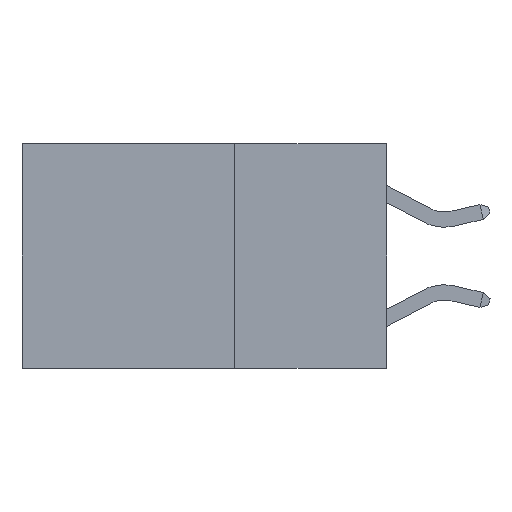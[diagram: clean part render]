
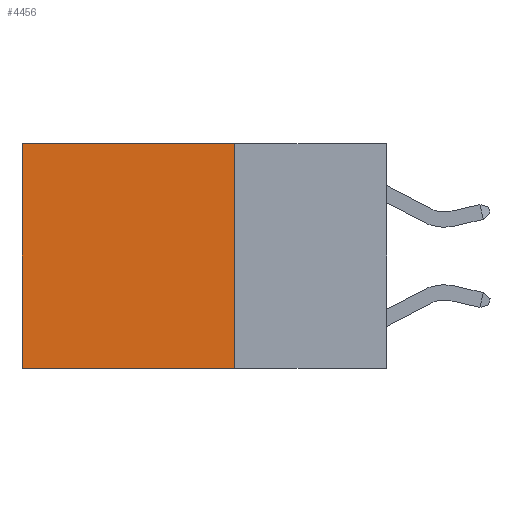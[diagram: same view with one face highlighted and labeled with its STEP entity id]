
A CAD part, left-side view. The second image highlights one B-rep face of the part: STEP entity #4456.
In plain terms, the highlighted planar face has unit normal (-1, 0, 0).
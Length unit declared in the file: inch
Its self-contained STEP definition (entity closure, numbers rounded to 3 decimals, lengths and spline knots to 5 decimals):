
#65 = LINE ( 'NONE', #5386, #7478 ) ;
#236 = CARTESIAN_POINT ( 'NONE',  ( 0.2625, 0.25, 0. ) ) ;
#237 = DIRECTION ( 'NONE',  ( 0., 1., 0. ) ) ;
#862 = PLANE ( 'NONE',  #7459 ) ;
#888 = VERTEX_POINT ( 'NONE', #8403 ) ;
#942 = CARTESIAN_POINT ( 'NONE',  ( 0.2625, 0.25, -0.37 ) ) ;
#1309 = LINE ( 'NONE', #7351, #4073 ) ;
#2309 = CARTESIAN_POINT ( 'NONE',  ( 0.2625, 0.25, 0. ) ) ;
#2523 = VECTOR ( 'NONE', #3492, 39.37008 ) ;
#2684 = FACE_OUTER_BOUND ( 'NONE', #4488, .T. ) ;
#2842 = EDGE_CURVE ( 'NONE', #2978, #7182, #1309, .T. ) ;
#2978 = VERTEX_POINT ( 'NONE', #942 ) ;
#3234 = VECTOR ( 'NONE', #237, 39.37008 ) ;
#3473 = DIRECTION ( 'NONE',  ( 0., 0., -1. ) ) ;
#3492 = DIRECTION ( 'NONE',  ( 0., 0., -1. ) ) ;
#3498 = EDGE_CURVE ( 'NONE', #4253, #2978, #65, .T. ) ;
#3987 = CARTESIAN_POINT ( 'NONE',  ( 0.2625, 0.25, 0. ) ) ;
#4073 = VECTOR ( 'NONE', #5890, 39.37008 ) ;
#4125 = DIRECTION ( 'NONE',  ( 0., 0., -1. ) ) ;
#4253 = VERTEX_POINT ( 'NONE', #236 ) ;
#4313 = ORIENTED_EDGE ( 'NONE', *, *, #6847, .T. ) ;
#4456 = ADVANCED_FACE ( 'NONE', ( #2684 ), #862, .F. ) ;
#4488 = EDGE_LOOP ( 'NONE', ( #4539, #7714, #7367, #4313 ) ) ;
#4539 = ORIENTED_EDGE ( 'NONE', *, *, #6703, .T. ) ;
#5284 = CARTESIAN_POINT ( 'NONE',  ( 0.2625, 0.6, 0. ) ) ;
#5386 = CARTESIAN_POINT ( 'NONE',  ( 0.2625, 0.25, 0. ) ) ;
#5890 = DIRECTION ( 'NONE',  ( 0., 1., 0. ) ) ;
#5920 = LINE ( 'NONE', #5284, #2523 ) ;
#6167 = LINE ( 'NONE', #2309, #3234 ) ;
#6703 = EDGE_CURVE ( 'NONE', #888, #7182, #5920, .T. ) ;
#6847 = EDGE_CURVE ( 'NONE', #4253, #888, #6167, .T. ) ;
#7182 = VERTEX_POINT ( 'NONE', #8043 ) ;
#7351 = CARTESIAN_POINT ( 'NONE',  ( 0.2625, 0.25, -0.37 ) ) ;
#7367 = ORIENTED_EDGE ( 'NONE', *, *, #3498, .F. ) ;
#7372 = DIRECTION ( 'NONE',  ( 1., 0., 0. ) ) ;
#7459 = AXIS2_PLACEMENT_3D ( 'NONE', #3987, #7372, #4125 ) ;
#7478 = VECTOR ( 'NONE', #3473, 39.37008 ) ;
#7714 = ORIENTED_EDGE ( 'NONE', *, *, #2842, .F. ) ;
#8043 = CARTESIAN_POINT ( 'NONE',  ( 0.2625, 0.6, -0.37 ) ) ;
#8403 = CARTESIAN_POINT ( 'NONE',  ( 0.2625, 0.6, 0. ) ) ;
